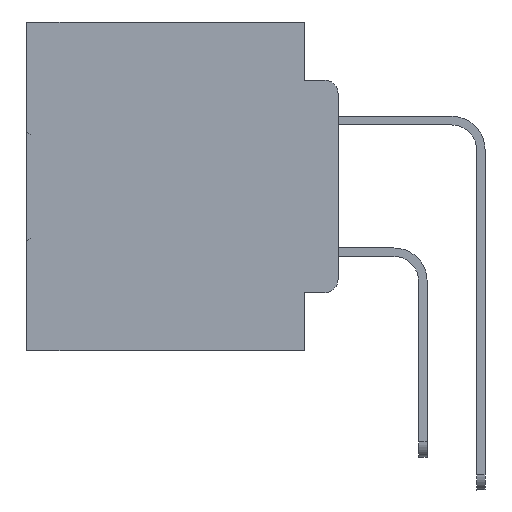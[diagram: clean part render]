
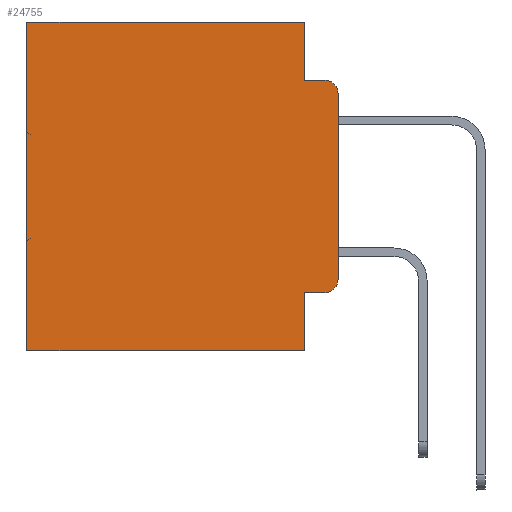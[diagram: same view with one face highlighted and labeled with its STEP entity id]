
A CAD part, left-side view. The second image highlights one B-rep face of the part: STEP entity #24755.
In plain terms, the highlighted planar face has unit normal (-1, 0, 0).
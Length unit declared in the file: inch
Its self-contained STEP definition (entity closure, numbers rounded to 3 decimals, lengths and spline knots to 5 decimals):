
#797 = CARTESIAN_POINT ( 'NONE',  ( 0.298, 0., -0.5 ) ) ;
#1137 = CARTESIAN_POINT ( 'NONE',  ( 0.298, 0.051, -0.4115 ) ) ;
#1244 = CIRCLE ( 'NONE', #30452, 0.02 ) ;
#1460 = EDGE_CURVE ( 'NONE', #10193, #29662, #23788, .T. ) ;
#1720 = AXIS2_PLACEMENT_3D ( 'NONE', #11240, #24895, #10225 ) ;
#2610 = CARTESIAN_POINT ( 'NONE',  ( 0.298, 0., -0.3915 ) ) ;
#3375 = LINE ( 'NONE', #9825, #12390 ) ;
#4030 = DIRECTION ( 'NONE',  ( 0., 1., 0. ) ) ;
#5043 = ORIENTED_EDGE ( 'NONE', *, *, #33922, .F. ) ;
#5717 = VECTOR ( 'NONE', #34081, 39.37008 ) ;
#5903 = ORIENTED_EDGE ( 'NONE', *, *, #11452, .F. ) ;
#6324 = DIRECTION ( 'NONE',  ( -1., 0., 0. ) ) ;
#9144 = ORIENTED_EDGE ( 'NONE', *, *, #34253, .F. ) ;
#9480 = DIRECTION ( 'NONE',  ( 0., 0., -1. ) ) ;
#9825 = CARTESIAN_POINT ( 'NONE',  ( 0.298, 0.051, 0. ) ) ;
#10193 = VERTEX_POINT ( 'NONE', #20816 ) ;
#10225 = DIRECTION ( 'NONE',  ( 0., 0., -1. ) ) ;
#10442 = FACE_OUTER_BOUND ( 'NONE', #25878, .T. ) ;
#10759 = ORIENTED_EDGE ( 'NONE', *, *, #34360, .T. ) ;
#11240 = CARTESIAN_POINT ( 'NONE',  ( 0.298, 0.02, -0.3915 ) ) ;
#11452 = EDGE_CURVE ( 'NONE', #28033, #32731, #20510, .T. ) ;
#11637 = CARTESIAN_POINT ( 'NONE',  ( 0.298, 0.051, -0.5 ) ) ;
#11829 = LINE ( 'NONE', #14532, #33873 ) ;
#12218 = VERTEX_POINT ( 'NONE', #24898 ) ;
#12390 = VECTOR ( 'NONE', #9480, 39.37008 ) ;
#12887 = ORIENTED_EDGE ( 'NONE', *, *, #1460, .F. ) ;
#12941 = CARTESIAN_POINT ( 'NONE',  ( 0.298, 0., 0. ) ) ;
#13912 = EDGE_CURVE ( 'NONE', #15553, #10193, #3375, .T. ) ;
#14115 = CARTESIAN_POINT ( 'NONE',  ( 0.298, 0.02, -0.0885 ) ) ;
#14532 = CARTESIAN_POINT ( 'NONE',  ( 0.298, 0.473, 0. ) ) ;
#14569 = DIRECTION ( 'NONE',  ( 0., 0., -1. ) ) ;
#14655 = LINE ( 'NONE', #22726, #25203 ) ;
#15128 = DIRECTION ( 'NONE',  ( 0., 0., -1. ) ) ;
#15268 = ORIENTED_EDGE ( 'NONE', *, *, #27109, .T. ) ;
#15553 = VERTEX_POINT ( 'NONE', #30792 ) ;
#15840 = LINE ( 'NONE', #24283, #32111 ) ;
#16262 = VERTEX_POINT ( 'NONE', #26957 ) ;
#17308 = VERTEX_POINT ( 'NONE', #2610 ) ;
#17343 = DIRECTION ( 'NONE',  ( 0., 0., -1. ) ) ;
#18920 = CIRCLE ( 'NONE', #1720, 0.02 ) ;
#20510 = LINE ( 'NONE', #797, #25933 ) ;
#20816 = CARTESIAN_POINT ( 'NONE',  ( 0.298, 0.051, -0.0885 ) ) ;
#21027 = EDGE_CURVE ( 'NONE', #12218, #32731, #11829, .T. ) ;
#21441 = VERTEX_POINT ( 'NONE', #33825 ) ;
#22546 = CARTESIAN_POINT ( 'NONE',  ( 0.298, 0.473, -0.5 ) ) ;
#22726 = CARTESIAN_POINT ( 'NONE',  ( 0.298, 0.051, 0. ) ) ;
#23029 = DIRECTION ( 'NONE',  ( 0., -1., 0. ) ) ;
#23366 = PLANE ( 'NONE',  #29993 ) ;
#23726 = VECTOR ( 'NONE', #32820, 39.37008 ) ;
#23788 = LINE ( 'NONE', #33716, #5717 ) ;
#23848 = EDGE_CURVE ( 'NONE', #15553, #12218, #26711, .T. ) ;
#24283 = CARTESIAN_POINT ( 'NONE',  ( 0.298, 0., 0. ) ) ;
#24755 = ADVANCED_FACE ( 'NONE', ( #10442 ), #23366, .F. ) ;
#24895 = DIRECTION ( 'NONE',  ( -1., 0., 0. ) ) ;
#24898 = CARTESIAN_POINT ( 'NONE',  ( 0.298, 0.473, 0. ) ) ;
#25203 = VECTOR ( 'NONE', #17343, 39.37008 ) ;
#25376 = LINE ( 'NONE', #1137, #27861 ) ;
#25520 = CARTESIAN_POINT ( 'NONE',  ( 0.298, 0.02, -0.1085 ) ) ;
#25878 = EDGE_LOOP ( 'NONE', ( #9144, #27727, #12887, #35083, #26447, #34216, #5903, #5043, #15268, #10759 ) ) ;
#25933 = VECTOR ( 'NONE', #4030, 39.37008 ) ;
#26447 = ORIENTED_EDGE ( 'NONE', *, *, #23848, .T. ) ;
#26711 = LINE ( 'NONE', #35177, #23726 ) ;
#26957 = CARTESIAN_POINT ( 'NONE',  ( 0.298, 0., -0.1085 ) ) ;
#26958 = DIRECTION ( 'NONE',  ( 0., 0., -1. ) ) ;
#27109 = EDGE_CURVE ( 'NONE', #21441, #32913, #25376, .T. ) ;
#27727 = ORIENTED_EDGE ( 'NONE', *, *, #32778, .T. ) ;
#27861 = VECTOR ( 'NONE', #23029, 39.37008 ) ;
#28033 = VERTEX_POINT ( 'NONE', #11637 ) ;
#28935 = DIRECTION ( 'NONE',  ( 1., 0., 0. ) ) ;
#29662 = VERTEX_POINT ( 'NONE', #14115 ) ;
#29993 = AXIS2_PLACEMENT_3D ( 'NONE', #12941, #28935, #15128 ) ;
#30452 = AXIS2_PLACEMENT_3D ( 'NONE', #25520, #6324, #14569 ) ;
#30792 = CARTESIAN_POINT ( 'NONE',  ( 0.298, 0.051, 0. ) ) ;
#32111 = VECTOR ( 'NONE', #26958, 39.37008 ) ;
#32731 = VERTEX_POINT ( 'NONE', #22546 ) ;
#32754 = CARTESIAN_POINT ( 'NONE',  ( 0.298, 0.02, -0.4115 ) ) ;
#32778 = EDGE_CURVE ( 'NONE', #16262, #29662, #1244, .T. ) ;
#32820 = DIRECTION ( 'NONE',  ( 0., 1., 0. ) ) ;
#32913 = VERTEX_POINT ( 'NONE', #32754 ) ;
#33716 = CARTESIAN_POINT ( 'NONE',  ( 0.298, 0.051, -0.0885 ) ) ;
#33825 = CARTESIAN_POINT ( 'NONE',  ( 0.298, 0.051, -0.4115 ) ) ;
#33873 = VECTOR ( 'NONE', #34087, 39.37008 ) ;
#33922 = EDGE_CURVE ( 'NONE', #21441, #28033, #14655, .T. ) ;
#34081 = DIRECTION ( 'NONE',  ( 0., -1., 0. ) ) ;
#34087 = DIRECTION ( 'NONE',  ( 0., 0., -1. ) ) ;
#34216 = ORIENTED_EDGE ( 'NONE', *, *, #21027, .T. ) ;
#34253 = EDGE_CURVE ( 'NONE', #16262, #17308, #15840, .T. ) ;
#34360 = EDGE_CURVE ( 'NONE', #32913, #17308, #18920, .T. ) ;
#35083 = ORIENTED_EDGE ( 'NONE', *, *, #13912, .F. ) ;
#35177 = CARTESIAN_POINT ( 'NONE',  ( 0.298, 0., 0. ) ) ;
